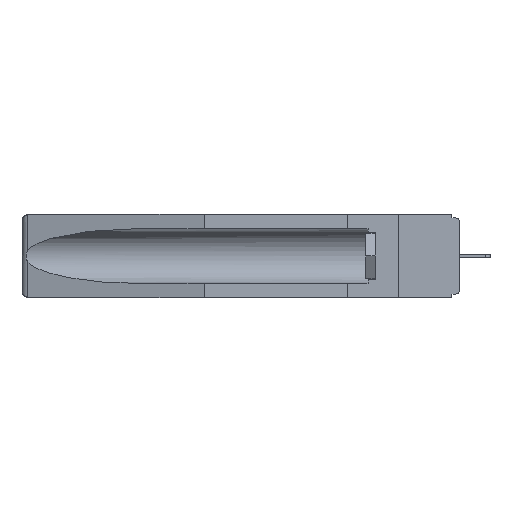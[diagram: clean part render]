
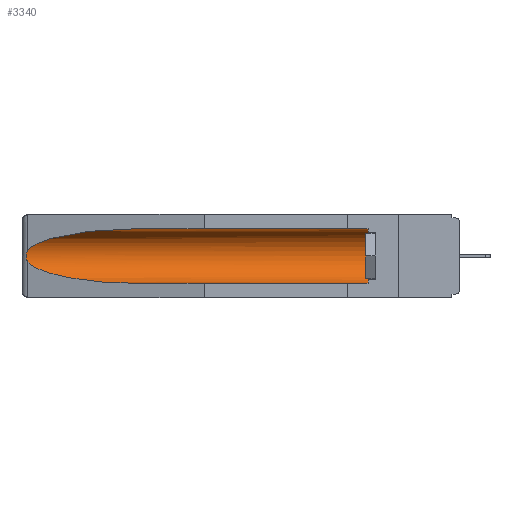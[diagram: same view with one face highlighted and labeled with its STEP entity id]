
A CAD part, left-side view. The second image highlights one B-rep face of the part: STEP entity #3340.
In plain terms, the highlighted cylindrical face has radius 2.857 mm (diameter 5.715 mm), a partial arc.
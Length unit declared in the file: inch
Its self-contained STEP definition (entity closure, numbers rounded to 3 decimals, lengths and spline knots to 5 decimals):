
#13 =( BOUNDED_CURVE ( )  B_SPLINE_CURVE ( 3, ( #2421, #1027, #12407, #10929 ),
 .UNSPECIFIED., .F., .F. ) 
 B_SPLINE_CURVE_WITH_KNOTS ( ( 4, 4 ),
 ( 0.1948, 1.5708 ),
 .UNSPECIFIED. ) 
 CURVE ( )  GEOMETRIC_REPRESENTATION_ITEM ( )  RATIONAL_B_SPLINE_CURVE ( ( 1., 0.848, 0.848, 1. ) ) 
 REPRESENTATION_ITEM ( '' )  );
#495 = DIRECTION ( 'NONE',  ( 0., 1., 0. ) ) ;
#580 = CARTESIAN_POINT ( 'NONE',  ( 0.26537, 1.52718, -0.19328 ) ) ;
#677 = CARTESIAN_POINT ( 'NONE',  ( 0.26655, 1.53094, -0.18657 ) ) ;
#879 = EDGE_CURVE ( 'NONE', #16875, #4486, #13, .T. ) ;
#1027 = CARTESIAN_POINT ( 'NONE',  ( 0.25451, 1.48313, -0.24835 ) ) ;
#1100 = CARTESIAN_POINT ( 'NONE',  ( 0.155, 1.07973, -0.059 ) ) ;
#1591 = VERTEX_POINT ( 'NONE', #17173 ) ;
#2042 = B_SPLINE_CURVE_WITH_KNOTS ( 'NONE', 3,
 ( #10490, #7521, #12054, #6397, #16291, #3643, #3366, #677, #9276, #580 ),
 .UNSPECIFIED., .F., .F.,
 ( 4, 2, 2, 2, 4 ),
 ( 0., 0.00029, 0.00058, 0.00087, 0.00117 ),
 .UNSPECIFIED. ) ;
#2421 = CARTESIAN_POINT ( 'NONE',  ( 0.26537, 1.52718, -0.19328 ) ) ;
#2600 = ORIENTED_EDGE ( 'NONE', *, *, #11860, .T. ) ;
#3340 = ADVANCED_FACE ( 'NONE', ( #6234 ), #15934, .F. ) ;
#3366 = CARTESIAN_POINT ( 'NONE',  ( 0.2673, 1.53269, -0.17917 ) ) ;
#3642 = CARTESIAN_POINT ( 'NONE',  ( 0.155, 1.07973, -0.059 ) ) ;
#3643 = CARTESIAN_POINT ( 'NONE',  ( 0.2675, 1.53308, -0.17534 ) ) ;
#4017 = EDGE_LOOP ( 'NONE', ( #13139, #4183, #8724, #12239, #2600, #13650 ) ) ;
#4183 = ORIENTED_EDGE ( 'NONE', *, *, #8190, .T. ) ;
#4486 = VERTEX_POINT ( 'NONE', #12028 ) ;
#4646 = EDGE_CURVE ( 'NONE', #17524, #1591, #16412, .T. ) ;
#5742 = CARTESIAN_POINT ( 'NONE',  ( 0.155, 0.126, -0.284 ) ) ;
#6234 = FACE_OUTER_BOUND ( 'NONE', #4017, .T. ) ;
#6397 = CARTESIAN_POINT ( 'NONE',  ( 0.2673, 1.5327, -0.16383 ) ) ;
#7015 = LINE ( 'NONE', #7115, #11719 ) ;
#7085 = CIRCLE ( 'NONE', #7387, 0.1125 ) ;
#7115 = CARTESIAN_POINT ( 'NONE',  ( 0.155, -0.30754, -0.059 ) ) ;
#7187 = CARTESIAN_POINT ( 'NONE',  ( 0.26537, 1.52718, -0.19328 ) ) ;
#7387 = AXIS2_PLACEMENT_3D ( 'NONE', #8298, #12547, #16876 ) ;
#7521 = CARTESIAN_POINT ( 'NONE',  ( 0.26597, 1.52961, -0.15275 ) ) ;
#7585 = LINE ( 'NONE', #10275, #8716 ) ;
#8052 = CARTESIAN_POINT ( 'NONE',  ( 0.25451, 1.48313, -0.09465 ) ) ;
#8190 = EDGE_CURVE ( 'NONE', #1591, #16875, #2042, .T. ) ;
#8298 = CARTESIAN_POINT ( 'NONE',  ( 0.155, 0.126, -0.1715 ) ) ;
#8716 = VECTOR ( 'NONE', #11851, 39.37008 ) ;
#8724 = ORIENTED_EDGE ( 'NONE', *, *, #879, .T. ) ;
#9019 = CARTESIAN_POINT ( 'NONE',  ( 0.155, -0.30754, -0.1715 ) ) ;
#9276 = CARTESIAN_POINT ( 'NONE',  ( 0.26597, 1.5296, -0.19026 ) ) ;
#10275 = CARTESIAN_POINT ( 'NONE',  ( 0.155, -0.30754, -0.284 ) ) ;
#10490 = CARTESIAN_POINT ( 'NONE',  ( 0.26537, 1.52718, -0.14972 ) ) ;
#10911 = CARTESIAN_POINT ( 'NONE',  ( 0.21114, 1.30732, -0.059 ) ) ;
#10929 = CARTESIAN_POINT ( 'NONE',  ( 0.155, 1.07973, -0.284 ) ) ;
#11719 = VECTOR ( 'NONE', #12851, 39.37008 ) ;
#11851 = DIRECTION ( 'NONE',  ( 0., 1., 0. ) ) ;
#11853 = VERTEX_POINT ( 'NONE', #15397 ) ;
#11860 = EDGE_CURVE ( 'NONE', #17638, #11853, #7085, .T. ) ;
#12028 = CARTESIAN_POINT ( 'NONE',  ( 0.155, 1.07973, -0.284 ) ) ;
#12054 = CARTESIAN_POINT ( 'NONE',  ( 0.26654, 1.53092, -0.15636 ) ) ;
#12239 = ORIENTED_EDGE ( 'NONE', *, *, #14386, .F. ) ;
#12407 = CARTESIAN_POINT ( 'NONE',  ( 0.21114, 1.30732, -0.284 ) ) ;
#12487 = CARTESIAN_POINT ( 'NONE',  ( 0.26537, 1.52718, -0.14972 ) ) ;
#12547 = DIRECTION ( 'NONE',  ( 0., -1., 0. ) ) ;
#12851 = DIRECTION ( 'NONE',  ( 0., 1., 0. ) ) ;
#13139 = ORIENTED_EDGE ( 'NONE', *, *, #4646, .T. ) ;
#13650 = ORIENTED_EDGE ( 'NONE', *, *, #15971, .T. ) ;
#13949 = AXIS2_PLACEMENT_3D ( 'NONE', #9019, #495, #15746 ) ;
#14386 = EDGE_CURVE ( 'NONE', #17638, #4486, #7585, .T. ) ;
#15397 = CARTESIAN_POINT ( 'NONE',  ( 0.155, 0.126, -0.059 ) ) ;
#15746 = DIRECTION ( 'NONE',  ( 0., 0., 1. ) ) ;
#15934 = CYLINDRICAL_SURFACE ( 'NONE', #13949, 0.1125 ) ;
#15971 = EDGE_CURVE ( 'NONE', #11853, #17524, #7015, .T. ) ;
#16291 = CARTESIAN_POINT ( 'NONE',  ( 0.2675, 1.53308, -0.16763 ) ) ;
#16412 =( BOUNDED_CURVE ( )  B_SPLINE_CURVE ( 3, ( #1100, #10911, #8052, #12487 ),
 .UNSPECIFIED., .F., .T. ) 
 B_SPLINE_CURVE_WITH_KNOTS ( ( 4, 4 ),
 ( 4.71239, 6.08839 ),
 .UNSPECIFIED. ) 
 CURVE ( )  GEOMETRIC_REPRESENTATION_ITEM ( )  RATIONAL_B_SPLINE_CURVE ( ( 1., 0.848, 0.848, 1. ) ) 
 REPRESENTATION_ITEM ( '' )  );
#16875 = VERTEX_POINT ( 'NONE', #7187 ) ;
#16876 = DIRECTION ( 'NONE',  ( 0., 0., 1. ) ) ;
#17173 = CARTESIAN_POINT ( 'NONE',  ( 0.26537, 1.52718, -0.14972 ) ) ;
#17524 = VERTEX_POINT ( 'NONE', #3642 ) ;
#17638 = VERTEX_POINT ( 'NONE', #5742 ) ;
